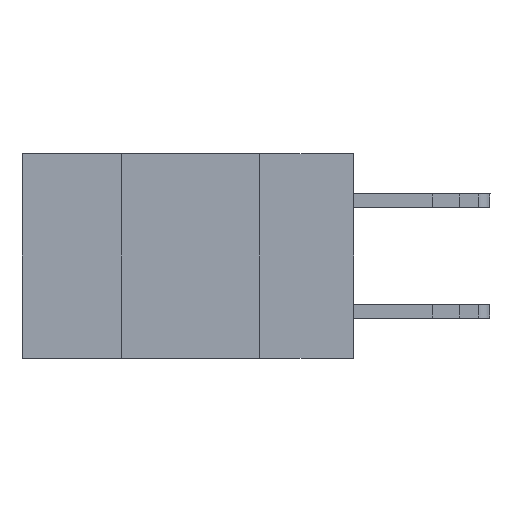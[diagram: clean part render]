
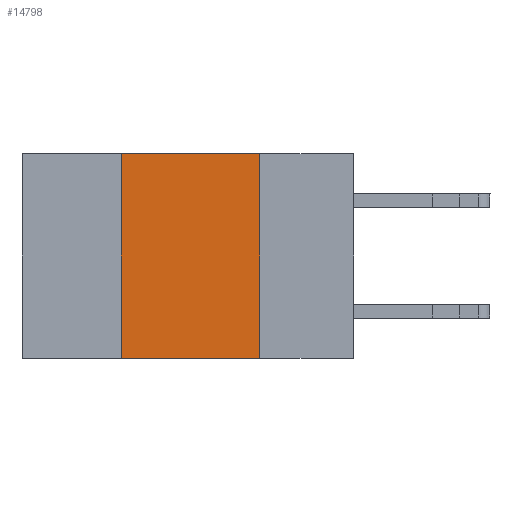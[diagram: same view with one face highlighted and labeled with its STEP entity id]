
A CAD part, left-side view. The second image highlights one B-rep face of the part: STEP entity #14798.
In plain terms, the highlighted planar face has unit normal (-1, 0, 0).
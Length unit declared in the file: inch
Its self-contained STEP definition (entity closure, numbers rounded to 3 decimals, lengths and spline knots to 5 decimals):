
#597 = CARTESIAN_POINT ( 'NONE',  ( 0., 0.17, -0.37 ) ) ;
#1079 = CARTESIAN_POINT ( 'NONE',  ( 0., 0.6, -0.37 ) ) ;
#1446 = EDGE_CURVE ( 'NONE', #11269, #13319, #7680, .T. ) ;
#1514 = DIRECTION ( 'NONE',  ( 1., 0., 0. ) ) ;
#1570 = ORIENTED_EDGE ( 'NONE', *, *, #12137, .F. ) ;
#1668 = CARTESIAN_POINT ( 'NONE',  ( 0., 0.6, 0. ) ) ;
#2274 = DIRECTION ( 'NONE',  ( 0., -1., 0. ) ) ;
#3854 = FACE_OUTER_BOUND ( 'NONE', #8979, .T. ) ;
#3886 = EDGE_CURVE ( 'NONE', #8516, #11269, #4745, .T. ) ;
#4020 = CARTESIAN_POINT ( 'NONE',  ( 0., 0.6, 0. ) ) ;
#4153 = ORIENTED_EDGE ( 'NONE', *, *, #1446, .F. ) ;
#4202 = CARTESIAN_POINT ( 'NONE',  ( 0., 0.17, 0. ) ) ;
#4745 = LINE ( 'NONE', #7133, #7455 ) ;
#4969 = CARTESIAN_POINT ( 'NONE',  ( 0., 0.17, 0. ) ) ;
#5075 = CARTESIAN_POINT ( 'NONE',  ( 0., 0.42, 0. ) ) ;
#6071 = DIRECTION ( 'NONE',  ( 0., 0., -1. ) ) ;
#6374 = VERTEX_POINT ( 'NONE', #597 ) ;
#7133 = CARTESIAN_POINT ( 'NONE',  ( 0., 0.42, 0. ) ) ;
#7305 = ORIENTED_EDGE ( 'NONE', *, *, #8364, .T. ) ;
#7313 = LINE ( 'NONE', #1079, #8395 ) ;
#7435 = PLANE ( 'NONE',  #8266 ) ;
#7455 = VECTOR ( 'NONE', #10872, 39.37008 ) ;
#7680 = LINE ( 'NONE', #1668, #12997 ) ;
#8266 = AXIS2_PLACEMENT_3D ( 'NONE', #4020, #1514, #13662 ) ;
#8364 = EDGE_CURVE ( 'NONE', #8516, #6374, #7313, .T. ) ;
#8395 = VECTOR ( 'NONE', #2274, 39.37008 ) ;
#8516 = VERTEX_POINT ( 'NONE', #14751 ) ;
#8979 = EDGE_LOOP ( 'NONE', ( #1570, #4153, #11797, #7305 ) ) ;
#10872 = DIRECTION ( 'NONE',  ( 0., 0., 1. ) ) ;
#11269 = VERTEX_POINT ( 'NONE', #5075 ) ;
#11290 = VECTOR ( 'NONE', #6071, 39.37008 ) ;
#11797 = ORIENTED_EDGE ( 'NONE', *, *, #3886, .F. ) ;
#12137 = EDGE_CURVE ( 'NONE', #13319, #6374, #12214, .T. ) ;
#12214 = LINE ( 'NONE', #4969, #11290 ) ;
#12997 = VECTOR ( 'NONE', #13980, 39.37008 ) ;
#13319 = VERTEX_POINT ( 'NONE', #4202 ) ;
#13662 = DIRECTION ( 'NONE',  ( 0., 0., -1. ) ) ;
#13980 = DIRECTION ( 'NONE',  ( 0., -1., 0. ) ) ;
#14751 = CARTESIAN_POINT ( 'NONE',  ( 0., 0.42, -0.37 ) ) ;
#14798 = ADVANCED_FACE ( 'NONE', ( #3854 ), #7435, .F. ) ;
